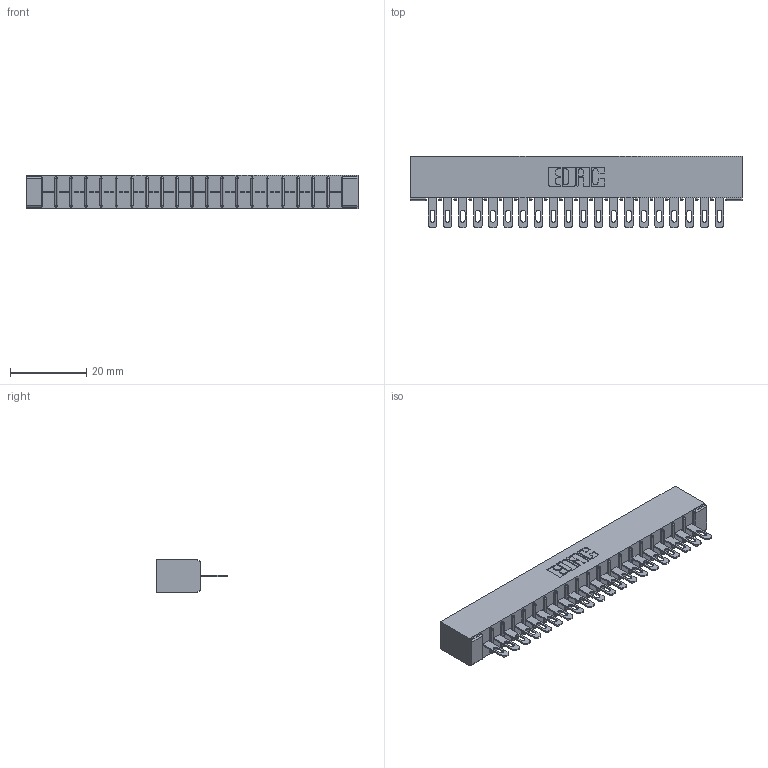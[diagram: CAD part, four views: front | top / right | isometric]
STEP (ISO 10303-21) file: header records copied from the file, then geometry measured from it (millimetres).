
FILE_DESCRIPTION (( 'STEP AP203' ), '1' );
FILE_NAME ('306-020-400-101.STEP', '2020-09-21T20:13:13', ( '' ), ( '' ), 'SwSTEP 2.0', 'SolidWorks 2020', '' );
FILE_SCHEMA (( 'CONFIG_CONTROL_DESIGN' ));
Length unit declared in the file: inch
Products named in the file (3): 306-290-001_100; 306-020-400-101; 306 Part_No Mounting
Assembly tree (21 placements, depth 2):
  306-020-400-101
    306 Part_No Mounting
    306-290-001_100  x20
Bounding box: 87.12 x 18.87 x 8.71 mm (x, y, z)
Volume: 6286.6 mm3; surface area: 9817.9 mm2
Topology: 21 solids, 21 shells, 1628 faces, 4592 edges, 2952 vertices
Faces by surface type: plane 1064, cylinder 484, sphere 80
Entity records: 21387 total; most frequent: CARTESIAN_POINT 3587, ORIENTED_EDGE 3552, DIRECTION 3540, EDGE_CURVE 1776, VECTOR 1378, LINE 1378, VERTEX_POINT 1128, AXIS2_PLACEMENT_3D 1081
